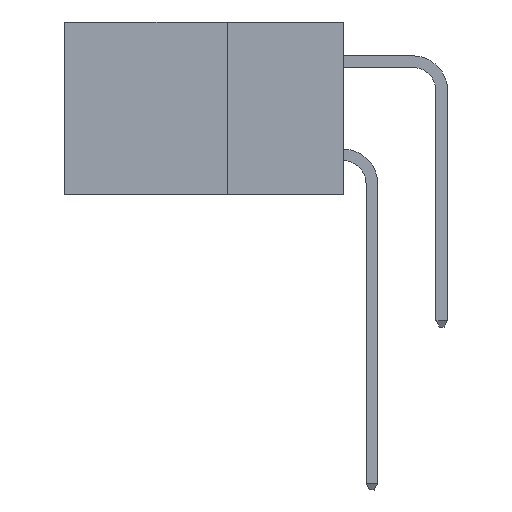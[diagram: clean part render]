
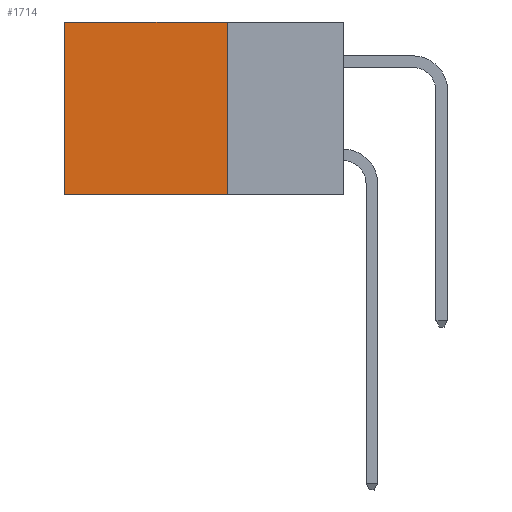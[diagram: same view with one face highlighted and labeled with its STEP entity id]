
A CAD part, left-side view. The second image highlights one B-rep face of the part: STEP entity #1714.
In plain terms, the highlighted planar face has unit normal (-1, 0, 0).
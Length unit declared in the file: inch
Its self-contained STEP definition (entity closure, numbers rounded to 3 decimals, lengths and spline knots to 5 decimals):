
#126 = ORIENTED_EDGE ( 'NONE', *, *, #10930, .F. ) ;
#1637 = DIRECTION ( 'NONE',  ( 0., 0., -1. ) ) ;
#1714 = ADVANCED_FACE ( 'NONE', ( #4695 ), #3764, .F. ) ;
#1777 = CARTESIAN_POINT ( 'NONE',  ( 0.298, 0.25, 0. ) ) ;
#2021 = CARTESIAN_POINT ( 'NONE',  ( 0.298, 0.25, -0.37 ) ) ;
#2330 = DIRECTION ( 'NONE',  ( 1., 0., 0. ) ) ;
#2737 = VERTEX_POINT ( 'NONE', #26890 ) ;
#2807 = VECTOR ( 'NONE', #28411, 39.37008 ) ;
#3764 = PLANE ( 'NONE',  #25573 ) ;
#4695 = FACE_OUTER_BOUND ( 'NONE', #16571, .T. ) ;
#5352 = CARTESIAN_POINT ( 'NONE',  ( 0.298, 0.25, 0. ) ) ;
#7576 = DIRECTION ( 'NONE',  ( 0., 0., -1. ) ) ;
#7598 = LINE ( 'NONE', #19047, #12739 ) ;
#7993 = CARTESIAN_POINT ( 'NONE',  ( 0.298, 0.25, 0. ) ) ;
#8709 = LINE ( 'NONE', #2021, #2807 ) ;
#9005 = VERTEX_POINT ( 'NONE', #1777 ) ;
#10184 = DIRECTION ( 'NONE',  ( 0., 0., -1. ) ) ;
#10190 = DIRECTION ( 'NONE',  ( 0., 1., 0. ) ) ;
#10930 = EDGE_CURVE ( 'NONE', #9005, #25904, #16478, .T. ) ;
#11332 = VECTOR ( 'NONE', #1637, 39.37008 ) ;
#12739 = VECTOR ( 'NONE', #10184, 39.37008 ) ;
#13893 = LINE ( 'NONE', #7993, #24931 ) ;
#14854 = CARTESIAN_POINT ( 'NONE',  ( 0.298, 0.25, 0. ) ) ;
#16478 = LINE ( 'NONE', #14854, #11332 ) ;
#16571 = EDGE_LOOP ( 'NONE', ( #19279, #27646, #126, #26659 ) ) ;
#17267 = VERTEX_POINT ( 'NONE', #28234 ) ;
#18006 = CARTESIAN_POINT ( 'NONE',  ( 0.298, 0.25, -0.37 ) ) ;
#19047 = CARTESIAN_POINT ( 'NONE',  ( 0.298, 0.6, 0. ) ) ;
#19279 = ORIENTED_EDGE ( 'NONE', *, *, #28183, .T. ) ;
#24931 = VECTOR ( 'NONE', #10190, 39.37008 ) ;
#25573 = AXIS2_PLACEMENT_3D ( 'NONE', #5352, #2330, #7576 ) ;
#25904 = VERTEX_POINT ( 'NONE', #18006 ) ;
#26183 = EDGE_CURVE ( 'NONE', #9005, #2737, #13893, .T. ) ;
#26659 = ORIENTED_EDGE ( 'NONE', *, *, #26183, .T. ) ;
#26890 = CARTESIAN_POINT ( 'NONE',  ( 0.298, 0.6, 0. ) ) ;
#27043 = EDGE_CURVE ( 'NONE', #25904, #17267, #8709, .T. ) ;
#27646 = ORIENTED_EDGE ( 'NONE', *, *, #27043, .F. ) ;
#28183 = EDGE_CURVE ( 'NONE', #2737, #17267, #7598, .T. ) ;
#28234 = CARTESIAN_POINT ( 'NONE',  ( 0.298, 0.6, -0.37 ) ) ;
#28411 = DIRECTION ( 'NONE',  ( 0., 1., 0. ) ) ;
